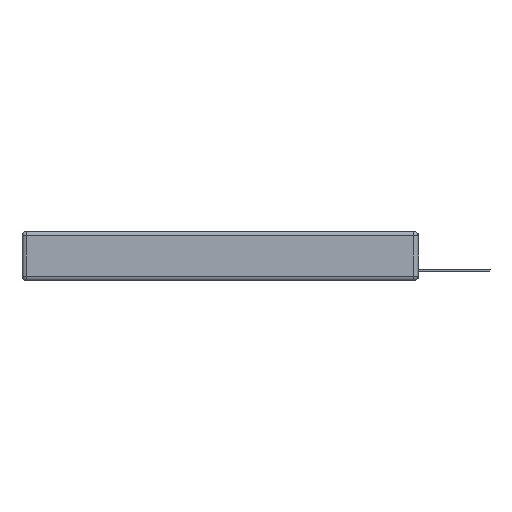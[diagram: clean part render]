
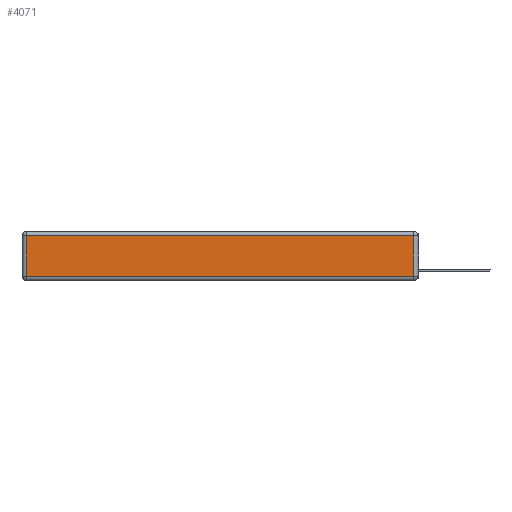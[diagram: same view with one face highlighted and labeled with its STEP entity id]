
A CAD part, left-side view. The second image highlights one B-rep face of the part: STEP entity #4071.
In plain terms, the highlighted planar face has unit normal (-1, 0, 0).
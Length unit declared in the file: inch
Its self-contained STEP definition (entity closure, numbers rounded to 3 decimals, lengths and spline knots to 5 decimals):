
#133 = EDGE_CURVE ( 'NONE', #14812, #15498, #4227, .T. ) ;
#1230 = FACE_OUTER_BOUND ( 'NONE', #9624, .T. ) ;
#1296 = VECTOR ( 'NONE', #9020, 39.37008 ) ;
#1561 = VERTEX_POINT ( 'NONE', #15106 ) ;
#1622 = VECTOR ( 'NONE', #12721, 39.37008 ) ;
#1938 = CARTESIAN_POINT ( 'NONE',  ( 0., 2.72, -0.343 ) ) ;
#3947 = LINE ( 'NONE', #15898, #1296 ) ;
#4071 = ADVANCED_FACE ( 'NONE', ( #1230 ), #10960, .T. ) ;
#4227 = LINE ( 'NONE', #13423, #4343 ) ;
#4343 = VECTOR ( 'NONE', #6623, 39.37008 ) ;
#5295 = ORIENTED_EDGE ( 'NONE', *, *, #133, .T. ) ;
#5302 = CARTESIAN_POINT ( 'NONE',  ( 0., 0., -0.343 ) ) ;
#6185 = LINE ( 'NONE', #1938, #1622 ) ;
#6623 = DIRECTION ( 'NONE',  ( 0., 0., 1. ) ) ;
#6968 = VERTEX_POINT ( 'NONE', #14179 ) ;
#7031 = ORIENTED_EDGE ( 'NONE', *, *, #12630, .T. ) ;
#7039 = VECTOR ( 'NONE', #15504, 39.37008 ) ;
#7922 = EDGE_CURVE ( 'NONE', #1561, #14812, #3947, .T. ) ;
#9020 = DIRECTION ( 'NONE',  ( 0., -1., 0. ) ) ;
#9322 = ORIENTED_EDGE ( 'NONE', *, *, #7922, .T. ) ;
#9583 = EDGE_CURVE ( 'NONE', #6968, #1561, #6185, .T. ) ;
#9624 = EDGE_LOOP ( 'NONE', ( #9322, #5295, #7031, #10316 ) ) ;
#9967 = CARTESIAN_POINT ( 'NONE',  ( 0., 0.03, -0.313 ) ) ;
#10109 = LINE ( 'NONE', #13831, #7039 ) ;
#10316 = ORIENTED_EDGE ( 'NONE', *, *, #9583, .T. ) ;
#10960 = PLANE ( 'NONE',  #14520 ) ;
#12630 = EDGE_CURVE ( 'NONE', #15498, #6968, #10109, .T. ) ;
#12721 = DIRECTION ( 'NONE',  ( 0., 0., -1. ) ) ;
#13423 = CARTESIAN_POINT ( 'NONE',  ( 0., 0.03, -0.343 ) ) ;
#13427 = DIRECTION ( 'NONE',  ( -1., 0., 0. ) ) ;
#13831 = CARTESIAN_POINT ( 'NONE',  ( 0., 2.75, -0.03 ) ) ;
#14179 = CARTESIAN_POINT ( 'NONE',  ( 0., 2.72, -0.03 ) ) ;
#14520 = AXIS2_PLACEMENT_3D ( 'NONE', #5302, #13427, #14752 ) ;
#14700 = CARTESIAN_POINT ( 'NONE',  ( 0., 0.03, -0.03 ) ) ;
#14752 = DIRECTION ( 'NONE',  ( 0., 0., 1. ) ) ;
#14812 = VERTEX_POINT ( 'NONE', #9967 ) ;
#15106 = CARTESIAN_POINT ( 'NONE',  ( 0., 2.72, -0.313 ) ) ;
#15498 = VERTEX_POINT ( 'NONE', #14700 ) ;
#15504 = DIRECTION ( 'NONE',  ( 0., 1., 0. ) ) ;
#15898 = CARTESIAN_POINT ( 'NONE',  ( 0., 0., -0.313 ) ) ;
